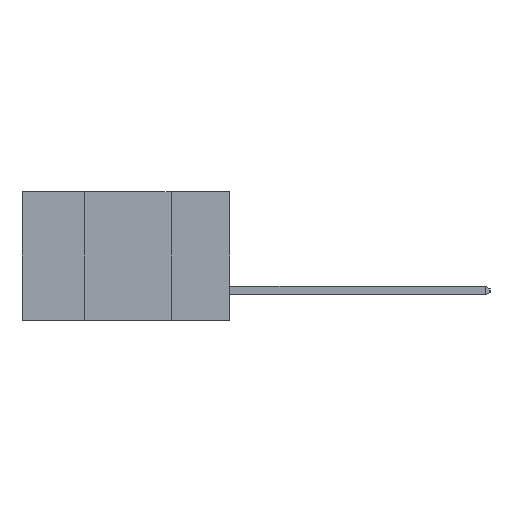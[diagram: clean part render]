
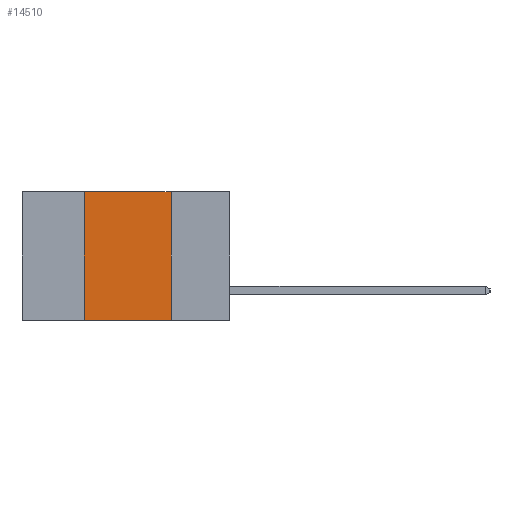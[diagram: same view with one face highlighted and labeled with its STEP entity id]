
A CAD part, left-side view. The second image highlights one B-rep face of the part: STEP entity #14510.
In plain terms, the highlighted planar face has unit normal (-1, 0, 0).
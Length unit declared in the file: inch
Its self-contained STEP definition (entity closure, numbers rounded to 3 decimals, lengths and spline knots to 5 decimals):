
#3 = PLANE ( 'NONE',  #22218 ) ;
#298 = VERTEX_POINT ( 'NONE', #26180 ) ;
#2078 = DIRECTION ( 'NONE',  ( 1., 0., 0. ) ) ;
#2314 = CARTESIAN_POINT ( 'NONE',  ( 0., 0.42, -0.37 ) ) ;
#2486 = VERTEX_POINT ( 'NONE', #2314 ) ;
#2667 = EDGE_LOOP ( 'NONE', ( #3349, #18325, #11397, #16177 ) ) ;
#2947 = VECTOR ( 'NONE', #5444, 39.37008 ) ;
#3349 = ORIENTED_EDGE ( 'NONE', *, *, #10023, .F. ) ;
#5444 = DIRECTION ( 'NONE',  ( 0., -1., 0. ) ) ;
#5706 = VERTEX_POINT ( 'NONE', #15573 ) ;
#6227 = LINE ( 'NONE', #25445, #17033 ) ;
#6323 = VECTOR ( 'NONE', #16068, 39.37008 ) ;
#7809 = DIRECTION ( 'NONE',  ( 0., -1., 0. ) ) ;
#8168 = VECTOR ( 'NONE', #7809, 39.37008 ) ;
#8316 = FACE_OUTER_BOUND ( 'NONE', #2667, .T. ) ;
#9038 = LINE ( 'NONE', #25558, #2947 ) ;
#10023 = EDGE_CURVE ( 'NONE', #298, #10083, #11747, .T. ) ;
#10083 = VERTEX_POINT ( 'NONE', #26151 ) ;
#11397 = ORIENTED_EDGE ( 'NONE', *, *, #12377, .F. ) ;
#11747 = LINE ( 'NONE', #24084, #6323 ) ;
#12377 = EDGE_CURVE ( 'NONE', #2486, #5706, #6227, .T. ) ;
#13416 = DIRECTION ( 'NONE',  ( 0., 0., 1. ) ) ;
#13639 = EDGE_CURVE ( 'NONE', #5706, #298, #9038, .T. ) ;
#14273 = CARTESIAN_POINT ( 'NONE',  ( 0., 0.6, 0. ) ) ;
#14510 = ADVANCED_FACE ( 'NONE', ( #8316 ), #3, .F. ) ;
#15573 = CARTESIAN_POINT ( 'NONE',  ( 0., 0.42, 0. ) ) ;
#16068 = DIRECTION ( 'NONE',  ( 0., 0., -1. ) ) ;
#16177 = ORIENTED_EDGE ( 'NONE', *, *, #19687, .T. ) ;
#16300 = DIRECTION ( 'NONE',  ( 0., 0., -1. ) ) ;
#17033 = VECTOR ( 'NONE', #13416, 39.37008 ) ;
#17690 = LINE ( 'NONE', #21965, #8168 ) ;
#18325 = ORIENTED_EDGE ( 'NONE', *, *, #13639, .F. ) ;
#19687 = EDGE_CURVE ( 'NONE', #2486, #10083, #17690, .T. ) ;
#21965 = CARTESIAN_POINT ( 'NONE',  ( 0., 0.6, -0.37 ) ) ;
#22218 = AXIS2_PLACEMENT_3D ( 'NONE', #14273, #2078, #16300 ) ;
#24084 = CARTESIAN_POINT ( 'NONE',  ( 0., 0.17, 0. ) ) ;
#25445 = CARTESIAN_POINT ( 'NONE',  ( 0., 0.42, 0. ) ) ;
#25558 = CARTESIAN_POINT ( 'NONE',  ( 0., 0.6, 0. ) ) ;
#26151 = CARTESIAN_POINT ( 'NONE',  ( 0., 0.17, -0.37 ) ) ;
#26180 = CARTESIAN_POINT ( 'NONE',  ( 0., 0.17, 0. ) ) ;
